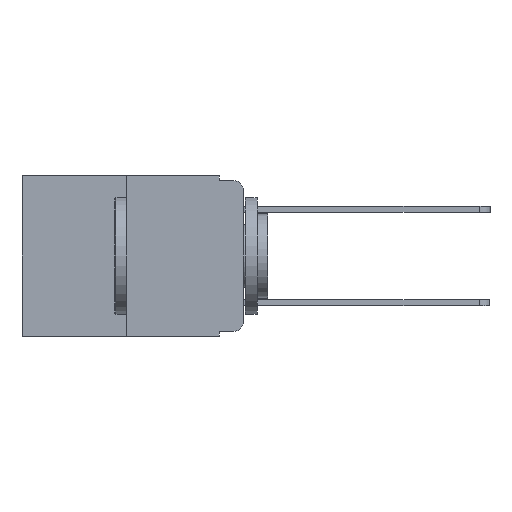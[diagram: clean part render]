
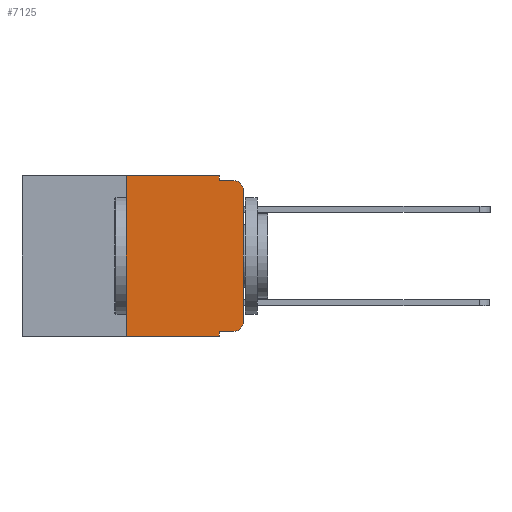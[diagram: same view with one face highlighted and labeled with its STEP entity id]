
A CAD part, left-side view. The second image highlights one B-rep face of the part: STEP entity #7125.
In plain terms, the highlighted planar face has unit normal (-1, 0, 0).
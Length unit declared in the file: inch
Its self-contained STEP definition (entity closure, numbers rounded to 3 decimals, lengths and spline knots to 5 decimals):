
#125 = ORIENTED_EDGE ( 'NONE', *, *, #13492, .F. ) ;
#229 = VERTEX_POINT ( 'NONE', #22953 ) ;
#358 = ORIENTED_EDGE ( 'NONE', *, *, #3409, .T. ) ;
#388 = EDGE_CURVE ( 'NONE', #10069, #5705, #17793, .T. ) ;
#439 = DIRECTION ( 'NONE',  ( 0., -1., 0. ) ) ;
#528 = VECTOR ( 'NONE', #12804, 39.37008 ) ;
#563 = ORIENTED_EDGE ( 'NONE', *, *, #9977, .T. ) ;
#1108 = EDGE_CURVE ( 'NONE', #1875, #10069, #22121, .T. ) ;
#1875 = VERTEX_POINT ( 'NONE', #13575 ) ;
#1985 = DIRECTION ( 'NONE',  ( 0., 0., 1. ) ) ;
#2631 = VERTEX_POINT ( 'NONE', #5294 ) ;
#2732 = VECTOR ( 'NONE', #13162, 39.37008 ) ;
#3409 = EDGE_CURVE ( 'NONE', #20077, #4305, #14565, .T. ) ;
#4003 = AXIS2_PLACEMENT_3D ( 'NONE', #17273, #6521, #19057 ) ;
#4256 = EDGE_CURVE ( 'NONE', #5705, #17146, #5555, .T. ) ;
#4305 = VERTEX_POINT ( 'NONE', #20068 ) ;
#4386 = VECTOR ( 'NONE', #439, 39.37008 ) ;
#5294 = CARTESIAN_POINT ( 'NONE',  ( 0., 0., -0.313 ) ) ;
#5478 = LINE ( 'NONE', #5995, #23293 ) ;
#5555 = LINE ( 'NONE', #22128, #4386 ) ;
#5556 = ORIENTED_EDGE ( 'NONE', *, *, #14548, .T. ) ;
#5627 = ORIENTED_EDGE ( 'NONE', *, *, #19354, .T. ) ;
#5705 = VERTEX_POINT ( 'NONE', #20632 ) ;
#5995 = CARTESIAN_POINT ( 'NONE',  ( 0., 0., 0. ) ) ;
#6262 = ORIENTED_EDGE ( 'NONE', *, *, #4256, .F. ) ;
#6521 = DIRECTION ( 'NONE',  ( -1., 0., 0. ) ) ;
#6587 = PLANE ( 'NONE',  #10574 ) ;
#6995 = VECTOR ( 'NONE', #19051, 39.37008 ) ;
#7125 = ADVANCED_FACE ( 'NONE', ( #11342 ), #6587, .F. ) ;
#7299 = DIRECTION ( 'NONE',  ( -1., 0., 0. ) ) ;
#7837 = DIRECTION ( 'NONE',  ( 0., 0., 1. ) ) ;
#7917 = CARTESIAN_POINT ( 'NONE',  ( 0., 0.473, 0. ) ) ;
#7974 = CIRCLE ( 'NONE', #13302, 0.02 ) ;
#8921 = LINE ( 'NONE', #9257, #17914 ) ;
#9257 = CARTESIAN_POINT ( 'NONE',  ( 0., 0.051, 0. ) ) ;
#9409 = CARTESIAN_POINT ( 'NONE',  ( 0., 0.051, -0.333 ) ) ;
#9442 = VERTEX_POINT ( 'NONE', #23362 ) ;
#9977 = EDGE_CURVE ( 'NONE', #4305, #2631, #7974, .T. ) ;
#10069 = VERTEX_POINT ( 'NONE', #20318 ) ;
#10165 = ORIENTED_EDGE ( 'NONE', *, *, #388, .F. ) ;
#10177 = DIRECTION ( 'NONE',  ( 0., 0., -1. ) ) ;
#10574 = AXIS2_PLACEMENT_3D ( 'NONE', #17262, #20878, #10177 ) ;
#10915 = CARTESIAN_POINT ( 'NONE',  ( 0., 0.02, -0.01 ) ) ;
#11022 = CARTESIAN_POINT ( 'NONE',  ( 0., 0.473, -0.343 ) ) ;
#11054 = DIRECTION ( 'NONE',  ( 0., 0., -1. ) ) ;
#11342 = FACE_OUTER_BOUND ( 'NONE', #16408, .T. ) ;
#11949 = ORIENTED_EDGE ( 'NONE', *, *, #1108, .F. ) ;
#12318 = EDGE_CURVE ( 'NONE', #9442, #229, #15153, .T. ) ;
#12466 = ORIENTED_EDGE ( 'NONE', *, *, #20059, .F. ) ;
#12670 = VECTOR ( 'NONE', #19582, 39.37008 ) ;
#12726 = ORIENTED_EDGE ( 'NONE', *, *, #12318, .T. ) ;
#12804 = DIRECTION ( 'NONE',  ( 0., -1., 0. ) ) ;
#12994 = CARTESIAN_POINT ( 'NONE',  ( 0., 0.051, -0.333 ) ) ;
#13162 = DIRECTION ( 'NONE',  ( 0., 0., -1. ) ) ;
#13302 = AXIS2_PLACEMENT_3D ( 'NONE', #18017, #7299, #19797 ) ;
#13480 = VECTOR ( 'NONE', #1985, 39.37008 ) ;
#13492 = EDGE_CURVE ( 'NONE', #20077, #229, #8921, .T. ) ;
#13575 = CARTESIAN_POINT ( 'NONE',  ( 0., 0.25, 0. ) ) ;
#14548 = EDGE_CURVE ( 'NONE', #2631, #15331, #5478, .T. ) ;
#14565 = LINE ( 'NONE', #9409, #6995 ) ;
#14765 = CARTESIAN_POINT ( 'NONE',  ( 0., 0.25, 0. ) ) ;
#15153 = LINE ( 'NONE', #11022, #528 ) ;
#15331 = VERTEX_POINT ( 'NONE', #20764 ) ;
#16408 = EDGE_LOOP ( 'NONE', ( #5556, #5627, #6262, #10165, #11949, #12466, #12726, #125, #358, #563 ) ) ;
#17146 = VERTEX_POINT ( 'NONE', #10915 ) ;
#17262 = CARTESIAN_POINT ( 'NONE',  ( 0., 0.473, 0. ) ) ;
#17273 = CARTESIAN_POINT ( 'NONE',  ( 0., 0.02, -0.03 ) ) ;
#17793 = LINE ( 'NONE', #22603, #2732 ) ;
#17914 = VECTOR ( 'NONE', #11054, 39.37008 ) ;
#18017 = CARTESIAN_POINT ( 'NONE',  ( 0., 0.02, -0.313 ) ) ;
#18254 = CIRCLE ( 'NONE', #4003, 0.02 ) ;
#19051 = DIRECTION ( 'NONE',  ( 0., -1., 0. ) ) ;
#19057 = DIRECTION ( 'NONE',  ( 0., 0., -1. ) ) ;
#19354 = EDGE_CURVE ( 'NONE', #15331, #17146, #18254, .T. ) ;
#19582 = DIRECTION ( 'NONE',  ( 0., -1., 0. ) ) ;
#19797 = DIRECTION ( 'NONE',  ( 0., 0., -1. ) ) ;
#20059 = EDGE_CURVE ( 'NONE', #9442, #1875, #22878, .T. ) ;
#20068 = CARTESIAN_POINT ( 'NONE',  ( 0., 0.02, -0.333 ) ) ;
#20077 = VERTEX_POINT ( 'NONE', #12994 ) ;
#20318 = CARTESIAN_POINT ( 'NONE',  ( 0., 0.051, 0. ) ) ;
#20632 = CARTESIAN_POINT ( 'NONE',  ( 0., 0.051, -0.01 ) ) ;
#20764 = CARTESIAN_POINT ( 'NONE',  ( 0., 0., -0.03 ) ) ;
#20878 = DIRECTION ( 'NONE',  ( 1., 0., 0. ) ) ;
#22121 = LINE ( 'NONE', #7917, #12670 ) ;
#22128 = CARTESIAN_POINT ( 'NONE',  ( 0., 0.051, -0.01 ) ) ;
#22603 = CARTESIAN_POINT ( 'NONE',  ( 0., 0.051, 0. ) ) ;
#22878 = LINE ( 'NONE', #14765, #13480 ) ;
#22953 = CARTESIAN_POINT ( 'NONE',  ( 0., 0.051, -0.343 ) ) ;
#23293 = VECTOR ( 'NONE', #7837, 39.37008 ) ;
#23362 = CARTESIAN_POINT ( 'NONE',  ( 0., 0.25, -0.343 ) ) ;
